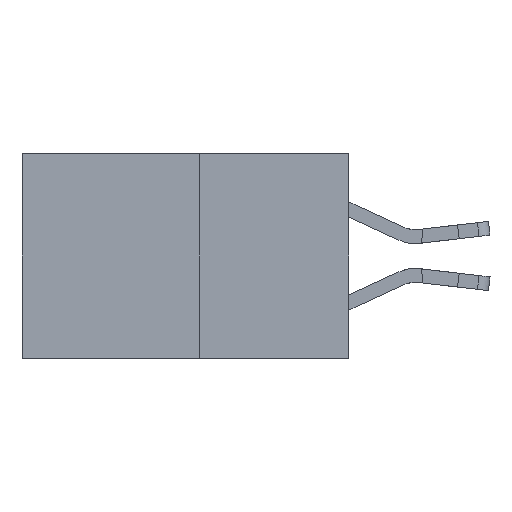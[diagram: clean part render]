
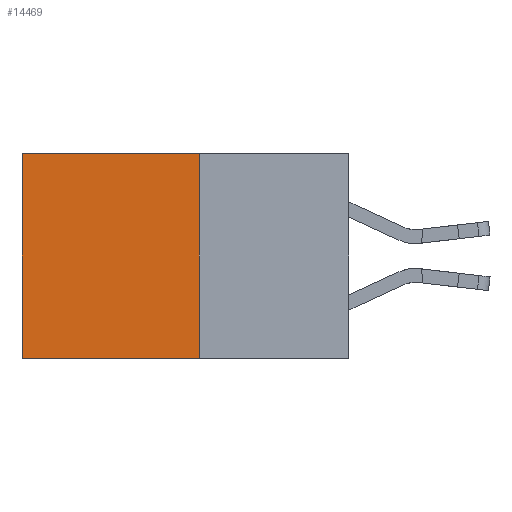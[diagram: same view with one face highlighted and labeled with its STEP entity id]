
A CAD part, left-side view. The second image highlights one B-rep face of the part: STEP entity #14469.
In plain terms, the highlighted planar face has unit normal (-1, 0, 0).
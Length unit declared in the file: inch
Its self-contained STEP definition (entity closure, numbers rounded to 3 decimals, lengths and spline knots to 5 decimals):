
#619 = DIRECTION ( 'NONE',  ( 0., 1., 0. ) ) ;
#1552 = EDGE_CURVE ( 'NONE', #13380, #4760, #4079, .T. ) ;
#2734 = CARTESIAN_POINT ( 'NONE',  ( 0.277, 0.59, -0.37 ) ) ;
#2960 = EDGE_CURVE ( 'NONE', #8466, #3342, #3805, .T. ) ;
#3239 = EDGE_CURVE ( 'NONE', #4760, #3342, #5626, .T. ) ;
#3342 = VERTEX_POINT ( 'NONE', #3369 ) ;
#3369 = CARTESIAN_POINT ( 'NONE',  ( 0.277, 0.59, -0.37 ) ) ;
#3386 = DIRECTION ( 'NONE',  ( 1., 0., 0. ) ) ;
#3805 = LINE ( 'NONE', #6970, #9629 ) ;
#4079 = LINE ( 'NONE', #5002, #12365 ) ;
#4760 = VERTEX_POINT ( 'NONE', #12892 ) ;
#5002 = CARTESIAN_POINT ( 'NONE',  ( 0.277, 0.27, 0. ) ) ;
#5215 = VECTOR ( 'NONE', #7853, 39.37008 ) ;
#5570 = ORIENTED_EDGE ( 'NONE', *, *, #1552, .T. ) ;
#5626 = LINE ( 'NONE', #2734, #5215 ) ;
#6970 = CARTESIAN_POINT ( 'NONE',  ( 0.277, 0.27, -0.37 ) ) ;
#7255 = EDGE_LOOP ( 'NONE', ( #8200, #7819, #9630, #5570 ) ) ;
#7713 = CARTESIAN_POINT ( 'NONE',  ( 0.277, 0.27, -0.37 ) ) ;
#7819 = ORIENTED_EDGE ( 'NONE', *, *, #2960, .F. ) ;
#7853 = DIRECTION ( 'NONE',  ( 0., 0., -1. ) ) ;
#8200 = ORIENTED_EDGE ( 'NONE', *, *, #3239, .T. ) ;
#8466 = VERTEX_POINT ( 'NONE', #7713 ) ;
#8894 = VECTOR ( 'NONE', #8907, 39.37008 ) ;
#8907 = DIRECTION ( 'NONE',  ( 0., 0., -1. ) ) ;
#9187 = CARTESIAN_POINT ( 'NONE',  ( 0.277, 0.27, 0. ) ) ;
#9629 = VECTOR ( 'NONE', #14068, 39.37008 ) ;
#9630 = ORIENTED_EDGE ( 'NONE', *, *, #11691, .F. ) ;
#10320 = PLANE ( 'NONE',  #13269 ) ;
#10321 = FACE_OUTER_BOUND ( 'NONE', #7255, .T. ) ;
#11422 = DIRECTION ( 'NONE',  ( 0., 0., -1. ) ) ;
#11490 = CARTESIAN_POINT ( 'NONE',  ( 0.277, 0.27, -0.37 ) ) ;
#11691 = EDGE_CURVE ( 'NONE', #13380, #8466, #11715, .T. ) ;
#11715 = LINE ( 'NONE', #11490, #8894 ) ;
#12365 = VECTOR ( 'NONE', #619, 39.37008 ) ;
#12892 = CARTESIAN_POINT ( 'NONE',  ( 0.277, 0.59, 0. ) ) ;
#13269 = AXIS2_PLACEMENT_3D ( 'NONE', #13460, #3386, #11422 ) ;
#13380 = VERTEX_POINT ( 'NONE', #9187 ) ;
#13460 = CARTESIAN_POINT ( 'NONE',  ( 0.277, 0.27, -0.37 ) ) ;
#14068 = DIRECTION ( 'NONE',  ( 0., 1., 0. ) ) ;
#14469 = ADVANCED_FACE ( 'NONE', ( #10321 ), #10320, .F. ) ;
